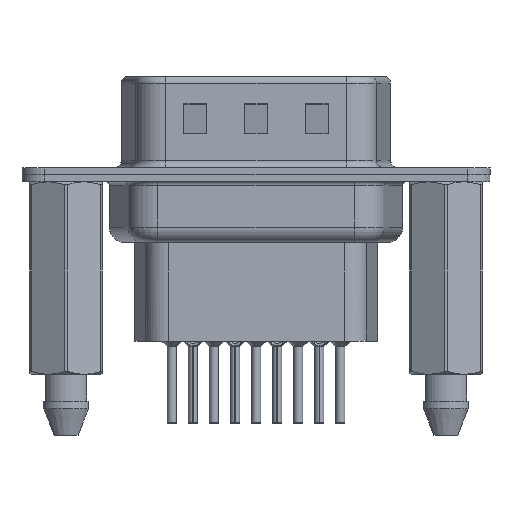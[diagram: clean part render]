
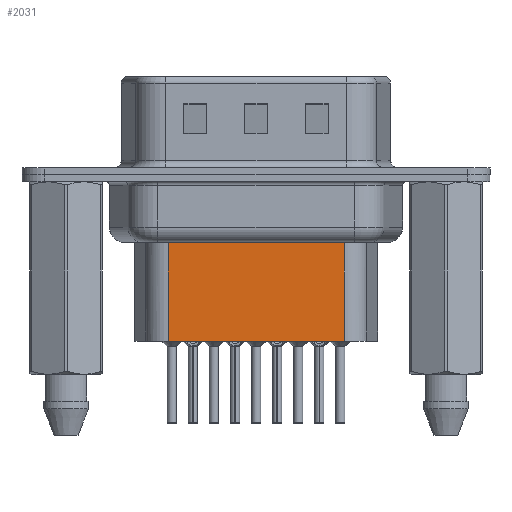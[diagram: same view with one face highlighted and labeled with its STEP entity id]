
A CAD part, front view. The second image highlights one B-rep face of the part: STEP entity #2031.
In plain terms, the highlighted planar face has unit normal (0, -1, 0).
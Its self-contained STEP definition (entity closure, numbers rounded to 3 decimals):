
#707 = LINE ( 'NONE', #7267, #13525 ) ;
#2031 = ADVANCED_FACE ( 'NONE', ( #11936 ), #15370, .T. ) ;
#2321 = VECTOR ( 'NONE', #4989, 1000. ) ;
#2866 = VECTOR ( 'NONE', #14998, 1000. ) ;
#4989 = DIRECTION ( 'NONE',  ( -1., 0., 0. ) ) ;
#5699 = DIRECTION ( 'NONE',  ( 1., 0., 0. ) ) ;
#6382 = DIRECTION ( 'NONE',  ( 0., 0., -1. ) ) ;
#7267 = CARTESIAN_POINT ( 'NONE',  ( 6.706, -3.5, -10.95 ) ) ;
#7479 = DIRECTION ( 'NONE',  ( -1., 0., 0. ) ) ;
#8194 = LINE ( 'NONE', #19512, #2321 ) ;
#8428 = LINE ( 'NONE', #13275, #2866 ) ;
#9018 = EDGE_LOOP ( 'NONE', ( #15342, #19838, #18349, #11448 ) ) ;
#9140 = CARTESIAN_POINT ( 'NONE',  ( 18.294, -3.5, -10.95 ) ) ;
#9445 = CARTESIAN_POINT ( 'NONE',  ( 18.294, -3.5, -4.097 ) ) ;
#9591 = EDGE_CURVE ( 'NONE', #13150, #14710, #8194, .T. ) ;
#9820 = LINE ( 'NONE', #14780, #20612 ) ;
#10430 = CARTESIAN_POINT ( 'NONE',  ( 6.706, -3.5, -3.1 ) ) ;
#10625 = EDGE_CURVE ( 'NONE', #14710, #18486, #9820, .T. ) ;
#11448 = ORIENTED_EDGE ( 'NONE', *, *, #18812, .F. ) ;
#11534 = VERTEX_POINT ( 'NONE', #9140 ) ;
#11936 = FACE_OUTER_BOUND ( 'NONE', #9018, .T. ) ;
#13150 = VERTEX_POINT ( 'NONE', #9445 ) ;
#13275 = CARTESIAN_POINT ( 'NONE',  ( 18.294, -3.5, -3.1 ) ) ;
#13525 = VECTOR ( 'NONE', #7479, 1000. ) ;
#14542 = CARTESIAN_POINT ( 'NONE',  ( 6.706, -3.5, -4.097 ) ) ;
#14710 = VERTEX_POINT ( 'NONE', #14542 ) ;
#14780 = CARTESIAN_POINT ( 'NONE',  ( 6.706, -3.5, -3.1 ) ) ;
#14998 = DIRECTION ( 'NONE',  ( 0., 0., -1. ) ) ;
#15342 = ORIENTED_EDGE ( 'NONE', *, *, #20260, .F. ) ;
#15370 = PLANE ( 'NONE',  #15867 ) ;
#15867 = AXIS2_PLACEMENT_3D ( 'NONE', #10430, #18729, #5699 ) ;
#15913 = CARTESIAN_POINT ( 'NONE',  ( 6.706, -3.5, -10.95 ) ) ;
#18349 = ORIENTED_EDGE ( 'NONE', *, *, #10625, .T. ) ;
#18486 = VERTEX_POINT ( 'NONE', #15913 ) ;
#18729 = DIRECTION ( 'NONE',  ( 0., -1., 0. ) ) ;
#18812 = EDGE_CURVE ( 'NONE', #11534, #18486, #707, .T. ) ;
#19512 = CARTESIAN_POINT ( 'NONE',  ( 6.459, -3.5, -4.097 ) ) ;
#19838 = ORIENTED_EDGE ( 'NONE', *, *, #9591, .T. ) ;
#20260 = EDGE_CURVE ( 'NONE', #13150, #11534, #8428, .T. ) ;
#20612 = VECTOR ( 'NONE', #6382, 1000. ) ;
